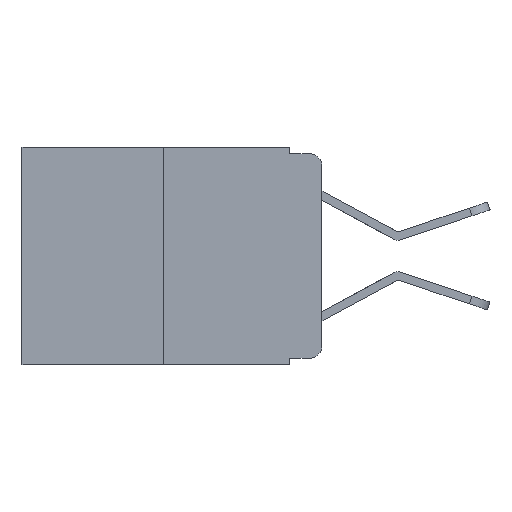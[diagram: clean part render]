
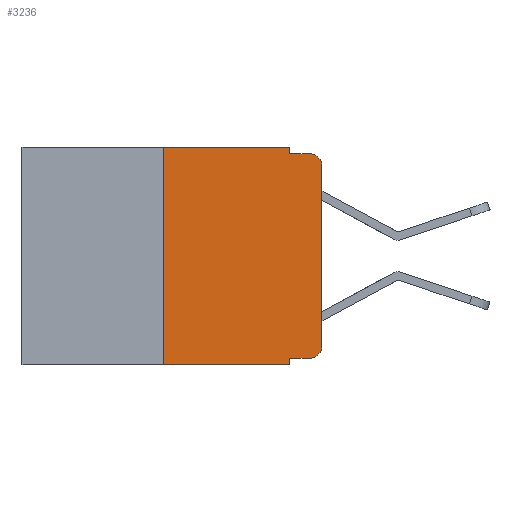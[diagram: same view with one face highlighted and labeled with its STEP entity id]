
A CAD part, left-side view. The second image highlights one B-rep face of the part: STEP entity #3236.
In plain terms, the highlighted planar face has unit normal (-1, 0, 0).
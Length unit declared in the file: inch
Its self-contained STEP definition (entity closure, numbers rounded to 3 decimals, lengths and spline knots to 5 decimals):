
#460 = DIRECTION ( 'NONE',  ( 0., 0., -1. ) ) ;
#467 = CARTESIAN_POINT ( 'NONE',  ( 0., 0., -0.313 ) ) ;
#564 = LINE ( 'NONE', #7563, #6659 ) ;
#621 = LINE ( 'NONE', #8976, #4826 ) ;
#915 = CARTESIAN_POINT ( 'NONE',  ( 0., 0.051, -0.333 ) ) ;
#1019 = VECTOR ( 'NONE', #6559, 39.37008 ) ;
#1179 = DIRECTION ( 'NONE',  ( 0., -1., 0. ) ) ;
#1181 = PLANE ( 'NONE',  #8650 ) ;
#1219 = DIRECTION ( 'NONE',  ( 0., 0., -1. ) ) ;
#1713 = CARTESIAN_POINT ( 'NONE',  ( 0., 0.25, -0.343 ) ) ;
#1822 = CARTESIAN_POINT ( 'NONE',  ( 0., 0.051, 0. ) ) ;
#1901 = EDGE_CURVE ( 'NONE', #9450, #4569, #5340, .T. ) ;
#1936 = DIRECTION ( 'NONE',  ( 0., -1., 0. ) ) ;
#1980 = EDGE_CURVE ( 'NONE', #3035, #2276, #621, .T. ) ;
#2067 = CARTESIAN_POINT ( 'NONE',  ( 0., 0.051, -0.333 ) ) ;
#2199 = CARTESIAN_POINT ( 'NONE',  ( 0., 0.051, -0.343 ) ) ;
#2276 = VERTEX_POINT ( 'NONE', #2199 ) ;
#2524 = VECTOR ( 'NONE', #1179, 39.37008 ) ;
#2603 = DIRECTION ( 'NONE',  ( -1., 0., 0. ) ) ;
#2781 = LINE ( 'NONE', #4538, #5021 ) ;
#2832 = DIRECTION ( 'NONE',  ( -1., 0., 0. ) ) ;
#2935 = CARTESIAN_POINT ( 'NONE',  ( 0., 0., 0. ) ) ;
#2992 = ORIENTED_EDGE ( 'NONE', *, *, #6490, .F. ) ;
#3035 = VERTEX_POINT ( 'NONE', #915 ) ;
#3134 = DIRECTION ( 'NONE',  ( 0., 0., -1. ) ) ;
#3146 = CARTESIAN_POINT ( 'NONE',  ( 0., 0.02, -0.01 ) ) ;
#3160 = ORIENTED_EDGE ( 'NONE', *, *, #3866, .T. ) ;
#3236 = ADVANCED_FACE ( 'NONE', ( #8834 ), #1181, .F. ) ;
#3408 = DIRECTION ( 'NONE',  ( 0., 0., -1. ) ) ;
#3466 = CARTESIAN_POINT ( 'NONE',  ( 0., 0.051, -0.01 ) ) ;
#3591 = VERTEX_POINT ( 'NONE', #4392 ) ;
#3631 = EDGE_CURVE ( 'NONE', #9890, #5050, #8702, .T. ) ;
#3826 = VECTOR ( 'NONE', #5722, 39.37008 ) ;
#3866 = EDGE_CURVE ( 'NONE', #6339, #2276, #2781, .T. ) ;
#3969 = ORIENTED_EDGE ( 'NONE', *, *, #9738, .T. ) ;
#3970 = VERTEX_POINT ( 'NONE', #9332 ) ;
#4073 = CARTESIAN_POINT ( 'NONE',  ( 0., 0.051, -0.01 ) ) ;
#4197 = AXIS2_PLACEMENT_3D ( 'NONE', #9251, #2603, #3134 ) ;
#4262 = ORIENTED_EDGE ( 'NONE', *, *, #1980, .F. ) ;
#4392 = CARTESIAN_POINT ( 'NONE',  ( 0., 0., -0.03 ) ) ;
#4538 = CARTESIAN_POINT ( 'NONE',  ( 0., 0.473, -0.343 ) ) ;
#4540 = ORIENTED_EDGE ( 'NONE', *, *, #1901, .F. ) ;
#4569 = VERTEX_POINT ( 'NONE', #3146 ) ;
#4614 = EDGE_CURVE ( 'NONE', #3970, #7146, #564, .T. ) ;
#4615 = EDGE_LOOP ( 'NONE', ( #10022, #4937, #4540, #7625, #8384, #2992, #3160, #4262, #3969, #5949 ) ) ;
#4826 = VECTOR ( 'NONE', #3408, 39.37008 ) ;
#4899 = EDGE_CURVE ( 'NONE', #7146, #9450, #10205, .T. ) ;
#4937 = ORIENTED_EDGE ( 'NONE', *, *, #6199, .T. ) ;
#5021 = VECTOR ( 'NONE', #6207, 39.37008 ) ;
#5050 = VERTEX_POINT ( 'NONE', #467 ) ;
#5297 = LINE ( 'NONE', #2067, #2524 ) ;
#5340 = LINE ( 'NONE', #3466, #9703 ) ;
#5482 = LINE ( 'NONE', #2935, #9131 ) ;
#5722 = DIRECTION ( 'NONE',  ( 0., 0., -1. ) ) ;
#5949 = ORIENTED_EDGE ( 'NONE', *, *, #3631, .T. ) ;
#6199 = EDGE_CURVE ( 'NONE', #3591, #4569, #7617, .T. ) ;
#6207 = DIRECTION ( 'NONE',  ( 0., -1., 0. ) ) ;
#6339 = VERTEX_POINT ( 'NONE', #1713 ) ;
#6490 = EDGE_CURVE ( 'NONE', #6339, #3970, #6621, .T. ) ;
#6559 = DIRECTION ( 'NONE',  ( 0., 0., 1. ) ) ;
#6621 = LINE ( 'NONE', #8193, #1019 ) ;
#6659 = VECTOR ( 'NONE', #9127, 39.37008 ) ;
#6674 = EDGE_CURVE ( 'NONE', #5050, #3591, #5482, .T. ) ;
#7028 = AXIS2_PLACEMENT_3D ( 'NONE', #9209, #2832, #460 ) ;
#7146 = VERTEX_POINT ( 'NONE', #1822 ) ;
#7464 = CARTESIAN_POINT ( 'NONE',  ( 0., 0.473, 0. ) ) ;
#7563 = CARTESIAN_POINT ( 'NONE',  ( 0., 0.473, 0. ) ) ;
#7617 = CIRCLE ( 'NONE', #4197, 0.02 ) ;
#7625 = ORIENTED_EDGE ( 'NONE', *, *, #4899, .F. ) ;
#7827 = CARTESIAN_POINT ( 'NONE',  ( 0., 0.02, -0.333 ) ) ;
#8181 = CARTESIAN_POINT ( 'NONE',  ( 0., 0.051, 0. ) ) ;
#8193 = CARTESIAN_POINT ( 'NONE',  ( 0., 0.25, 0. ) ) ;
#8384 = ORIENTED_EDGE ( 'NONE', *, *, #4614, .F. ) ;
#8545 = DIRECTION ( 'NONE',  ( 0., 0., 1. ) ) ;
#8650 = AXIS2_PLACEMENT_3D ( 'NONE', #7464, #9077, #1219 ) ;
#8702 = CIRCLE ( 'NONE', #7028, 0.02 ) ;
#8834 = FACE_OUTER_BOUND ( 'NONE', #4615, .T. ) ;
#8976 = CARTESIAN_POINT ( 'NONE',  ( 0., 0.051, 0. ) ) ;
#9077 = DIRECTION ( 'NONE',  ( 1., 0., 0. ) ) ;
#9127 = DIRECTION ( 'NONE',  ( 0., -1., 0. ) ) ;
#9131 = VECTOR ( 'NONE', #8545, 39.37008 ) ;
#9209 = CARTESIAN_POINT ( 'NONE',  ( 0., 0.02, -0.313 ) ) ;
#9251 = CARTESIAN_POINT ( 'NONE',  ( 0., 0.02, -0.03 ) ) ;
#9332 = CARTESIAN_POINT ( 'NONE',  ( 0., 0.25, 0. ) ) ;
#9450 = VERTEX_POINT ( 'NONE', #4073 ) ;
#9703 = VECTOR ( 'NONE', #1936, 39.37008 ) ;
#9738 = EDGE_CURVE ( 'NONE', #3035, #9890, #5297, .T. ) ;
#9890 = VERTEX_POINT ( 'NONE', #7827 ) ;
#10022 = ORIENTED_EDGE ( 'NONE', *, *, #6674, .T. ) ;
#10205 = LINE ( 'NONE', #8181, #3826 ) ;
